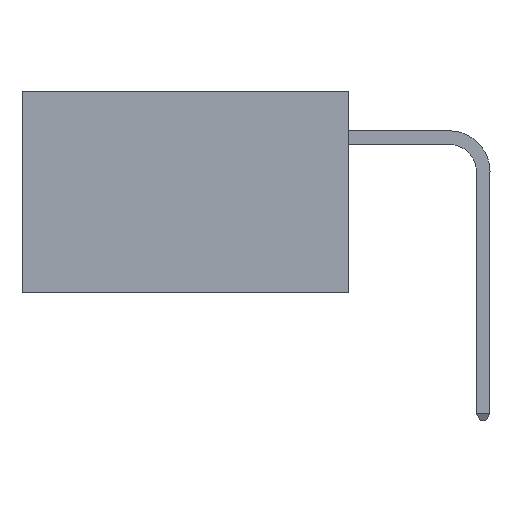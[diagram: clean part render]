
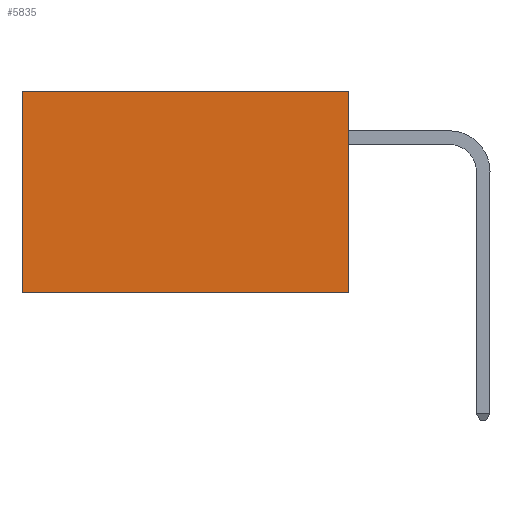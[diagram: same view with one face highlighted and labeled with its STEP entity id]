
A CAD part, left-side view. The second image highlights one B-rep face of the part: STEP entity #5835.
In plain terms, the highlighted planar face has unit normal (-1, 0, 0).
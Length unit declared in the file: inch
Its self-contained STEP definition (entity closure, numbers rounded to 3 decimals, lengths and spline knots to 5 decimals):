
#272 = EDGE_CURVE ( 'NONE', #7281, #3036, #3547, .T. ) ;
#1318 = EDGE_CURVE ( 'NONE', #1330, #3036, #6505, .T. ) ;
#1330 = VERTEX_POINT ( 'NONE', #5249 ) ;
#1550 = VECTOR ( 'NONE', #6281, 39.37008 ) ;
#1577 = EDGE_CURVE ( 'NONE', #9633, #1330, #4284, .T. ) ;
#1886 = LINE ( 'NONE', #9319, #3853 ) ;
#2081 = VECTOR ( 'NONE', #3166, 39.37008 ) ;
#2085 = FACE_OUTER_BOUND ( 'NONE', #2885, .T. ) ;
#2394 = CARTESIAN_POINT ( 'NONE',  ( 0.2875, 0.6, 0. ) ) ;
#2583 = ORIENTED_EDGE ( 'NONE', *, *, #1318, .F. ) ;
#2885 = EDGE_LOOP ( 'NONE', ( #8716, #2583, #9096, #6845 ) ) ;
#3036 = VERTEX_POINT ( 'NONE', #9145 ) ;
#3166 = DIRECTION ( 'NONE',  ( 0., 0., -1. ) ) ;
#3547 = LINE ( 'NONE', #6434, #1550 ) ;
#3853 = VECTOR ( 'NONE', #10072, 39.37008 ) ;
#4218 = AXIS2_PLACEMENT_3D ( 'NONE', #5650, #5466, #4231 ) ;
#4231 = DIRECTION ( 'NONE',  ( 0., 0., -1. ) ) ;
#4284 = LINE ( 'NONE', #4992, #2081 ) ;
#4992 = CARTESIAN_POINT ( 'NONE',  ( 0.2875, 0., 0. ) ) ;
#5249 = CARTESIAN_POINT ( 'NONE',  ( 0.2875, 0., -0.37 ) ) ;
#5260 = DIRECTION ( 'NONE',  ( 0., 1., 0. ) ) ;
#5304 = CARTESIAN_POINT ( 'NONE',  ( 0.2875, 0., -0.37 ) ) ;
#5464 = CARTESIAN_POINT ( 'NONE',  ( 0.2875, 0., 0. ) ) ;
#5466 = DIRECTION ( 'NONE',  ( 1., 0., 0. ) ) ;
#5650 = CARTESIAN_POINT ( 'NONE',  ( 0.2875, 0., 0. ) ) ;
#5835 = ADVANCED_FACE ( 'NONE', ( #2085 ), #8455, .F. ) ;
#6281 = DIRECTION ( 'NONE',  ( 0., 0., -1. ) ) ;
#6434 = CARTESIAN_POINT ( 'NONE',  ( 0.2875, 0.6, 0. ) ) ;
#6505 = LINE ( 'NONE', #5304, #10400 ) ;
#6845 = ORIENTED_EDGE ( 'NONE', *, *, #8946, .T. ) ;
#7281 = VERTEX_POINT ( 'NONE', #2394 ) ;
#8455 = PLANE ( 'NONE',  #4218 ) ;
#8716 = ORIENTED_EDGE ( 'NONE', *, *, #272, .T. ) ;
#8946 = EDGE_CURVE ( 'NONE', #9633, #7281, #1886, .T. ) ;
#9096 = ORIENTED_EDGE ( 'NONE', *, *, #1577, .F. ) ;
#9145 = CARTESIAN_POINT ( 'NONE',  ( 0.2875, 0.6, -0.37 ) ) ;
#9319 = CARTESIAN_POINT ( 'NONE',  ( 0.2875, 0., 0. ) ) ;
#9633 = VERTEX_POINT ( 'NONE', #5464 ) ;
#10072 = DIRECTION ( 'NONE',  ( 0., 1., 0. ) ) ;
#10400 = VECTOR ( 'NONE', #5260, 39.37008 ) ;
